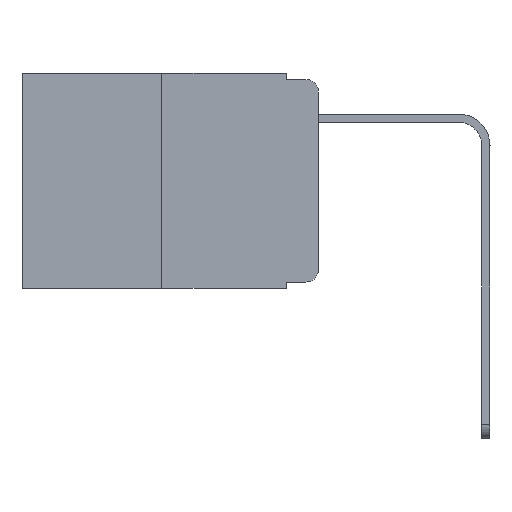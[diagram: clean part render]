
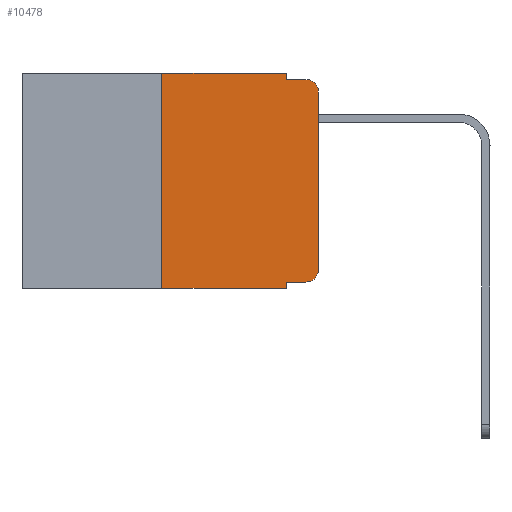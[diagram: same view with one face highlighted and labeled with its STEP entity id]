
A CAD part, left-side view. The second image highlights one B-rep face of the part: STEP entity #10478.
In plain terms, the highlighted planar face has unit normal (-1, 0, 0).
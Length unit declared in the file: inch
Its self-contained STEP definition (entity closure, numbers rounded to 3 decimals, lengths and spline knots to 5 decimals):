
#91 = VERTEX_POINT ( 'NONE', #7067 ) ;
#292 = CARTESIAN_POINT ( 'NONE',  ( 0., 0.25, 0. ) ) ;
#406 = LINE ( 'NONE', #9461, #6732 ) ;
#612 = DIRECTION ( 'NONE',  ( 0., -1., 0. ) ) ;
#641 = ORIENTED_EDGE ( 'NONE', *, *, #7964, .F. ) ;
#962 = EDGE_CURVE ( 'NONE', #13038, #2491, #13460, .T. ) ;
#1041 = EDGE_CURVE ( 'NONE', #91, #13038, #13301, .T. ) ;
#1203 = DIRECTION ( 'NONE',  ( 0., 0., 1. ) ) ;
#1241 = VECTOR ( 'NONE', #11664, 39.37008 ) ;
#1297 = DIRECTION ( 'NONE',  ( 0., 0., -1. ) ) ;
#1613 = VECTOR ( 'NONE', #12082, 39.37008 ) ;
#1673 = ORIENTED_EDGE ( 'NONE', *, *, #12184, .T. ) ;
#1841 = VERTEX_POINT ( 'NONE', #10940 ) ;
#2083 = LINE ( 'NONE', #6986, #6258 ) ;
#2445 = VERTEX_POINT ( 'NONE', #3387 ) ;
#2490 = DIRECTION ( 'NONE',  ( 0., 0., -1. ) ) ;
#2491 = VERTEX_POINT ( 'NONE', #6787 ) ;
#2557 = CARTESIAN_POINT ( 'NONE',  ( 0., 0.02, -0.333 ) ) ;
#2802 = VECTOR ( 'NONE', #5198, 39.37008 ) ;
#2973 = CARTESIAN_POINT ( 'NONE',  ( 0., 0.051, 0. ) ) ;
#3045 = ORIENTED_EDGE ( 'NONE', *, *, #10489, .T. ) ;
#3101 = VECTOR ( 'NONE', #2490, 39.37008 ) ;
#3387 = CARTESIAN_POINT ( 'NONE',  ( 0., 0.051, -0.343 ) ) ;
#3602 = ORIENTED_EDGE ( 'NONE', *, *, #13327, .T. ) ;
#3613 = CIRCLE ( 'NONE', #4885, 0.02 ) ;
#3756 = VECTOR ( 'NONE', #10365, 39.37008 ) ;
#4124 = DIRECTION ( 'NONE',  ( 0., 0., 1. ) ) ;
#4350 = ORIENTED_EDGE ( 'NONE', *, *, #962, .F. ) ;
#4607 = DIRECTION ( 'NONE',  ( -1., 0., 0. ) ) ;
#4625 = AXIS2_PLACEMENT_3D ( 'NONE', #11057, #11157, #7944 ) ;
#4651 = CARTESIAN_POINT ( 'NONE',  ( 0., 0.25, 0. ) ) ;
#4885 = AXIS2_PLACEMENT_3D ( 'NONE', #7748, #10828, #1297 ) ;
#5175 = VERTEX_POINT ( 'NONE', #2557 ) ;
#5198 = DIRECTION ( 'NONE',  ( 0., -1., 0. ) ) ;
#5305 = VERTEX_POINT ( 'NONE', #8576 ) ;
#5349 = VERTEX_POINT ( 'NONE', #10925 ) ;
#5919 = CARTESIAN_POINT ( 'NONE',  ( 0., 0., -0.313 ) ) ;
#5934 = LINE ( 'NONE', #8931, #1613 ) ;
#6072 = AXIS2_PLACEMENT_3D ( 'NONE', #13096, #4607, #12996 ) ;
#6258 = VECTOR ( 'NONE', #612, 39.37008 ) ;
#6732 = VECTOR ( 'NONE', #4124, 39.37008 ) ;
#6758 = CARTESIAN_POINT ( 'NONE',  ( 0., 0.051, -0.01 ) ) ;
#6787 = CARTESIAN_POINT ( 'NONE',  ( 0., 0.051, 0. ) ) ;
#6897 = ORIENTED_EDGE ( 'NONE', *, *, #10337, .T. ) ;
#6986 = CARTESIAN_POINT ( 'NONE',  ( 0., 0.473, -0.343 ) ) ;
#7067 = CARTESIAN_POINT ( 'NONE',  ( 0., 0.25, -0.343 ) ) ;
#7298 = FACE_OUTER_BOUND ( 'NONE', #13647, .T. ) ;
#7341 = CARTESIAN_POINT ( 'NONE',  ( 0., 0.051, -0.01 ) ) ;
#7595 = CIRCLE ( 'NONE', #6072, 0.02 ) ;
#7690 = EDGE_CURVE ( 'NONE', #10163, #5305, #11460, .T. ) ;
#7748 = CARTESIAN_POINT ( 'NONE',  ( 0., 0.02, -0.313 ) ) ;
#7944 = DIRECTION ( 'NONE',  ( 0., 0., -1. ) ) ;
#7964 = EDGE_CURVE ( 'NONE', #1841, #2445, #13416, .T. ) ;
#8316 = EDGE_CURVE ( 'NONE', #91, #2445, #2083, .T. ) ;
#8576 = CARTESIAN_POINT ( 'NONE',  ( 0., 0.02, -0.01 ) ) ;
#8931 = CARTESIAN_POINT ( 'NONE',  ( 0., 0.051, -0.333 ) ) ;
#8974 = PLANE ( 'NONE',  #4625 ) ;
#9461 = CARTESIAN_POINT ( 'NONE',  ( 0., 0., 0. ) ) ;
#9640 = VERTEX_POINT ( 'NONE', #5919 ) ;
#10100 = ORIENTED_EDGE ( 'NONE', *, *, #7690, .F. ) ;
#10163 = VERTEX_POINT ( 'NONE', #6758 ) ;
#10337 = EDGE_CURVE ( 'NONE', #5175, #9640, #3613, .T. ) ;
#10365 = DIRECTION ( 'NONE',  ( 0., -1., 0. ) ) ;
#10478 = ADVANCED_FACE ( 'NONE', ( #7298 ), #8974, .F. ) ;
#10489 = EDGE_CURVE ( 'NONE', #1841, #5175, #5934, .T. ) ;
#10496 = VECTOR ( 'NONE', #1203, 39.37008 ) ;
#10828 = DIRECTION ( 'NONE',  ( -1., 0., 0. ) ) ;
#10925 = CARTESIAN_POINT ( 'NONE',  ( 0., 0., -0.03 ) ) ;
#10932 = CARTESIAN_POINT ( 'NONE',  ( 0., 0.051, 0. ) ) ;
#10940 = CARTESIAN_POINT ( 'NONE',  ( 0., 0.051, -0.333 ) ) ;
#11057 = CARTESIAN_POINT ( 'NONE',  ( 0., 0.473, 0. ) ) ;
#11157 = DIRECTION ( 'NONE',  ( 1., 0., 0. ) ) ;
#11460 = LINE ( 'NONE', #7341, #3756 ) ;
#11628 = ORIENTED_EDGE ( 'NONE', *, *, #8316, .T. ) ;
#11629 = CARTESIAN_POINT ( 'NONE',  ( 0., 0.473, 0. ) ) ;
#11664 = DIRECTION ( 'NONE',  ( 0., 0., -1. ) ) ;
#12082 = DIRECTION ( 'NONE',  ( 0., -1., 0. ) ) ;
#12184 = EDGE_CURVE ( 'NONE', #9640, #5349, #406, .T. ) ;
#12409 = LINE ( 'NONE', #2973, #1241 ) ;
#12996 = DIRECTION ( 'NONE',  ( 0., 0., -1. ) ) ;
#13038 = VERTEX_POINT ( 'NONE', #4651 ) ;
#13096 = CARTESIAN_POINT ( 'NONE',  ( 0., 0.02, -0.03 ) ) ;
#13298 = ORIENTED_EDGE ( 'NONE', *, *, #13728, .F. ) ;
#13301 = LINE ( 'NONE', #292, #10496 ) ;
#13327 = EDGE_CURVE ( 'NONE', #5349, #5305, #7595, .T. ) ;
#13344 = ORIENTED_EDGE ( 'NONE', *, *, #1041, .F. ) ;
#13416 = LINE ( 'NONE', #10932, #3101 ) ;
#13460 = LINE ( 'NONE', #11629, #2802 ) ;
#13647 = EDGE_LOOP ( 'NONE', ( #1673, #3602, #10100, #13298, #4350, #13344, #11628, #641, #3045, #6897 ) ) ;
#13728 = EDGE_CURVE ( 'NONE', #2491, #10163, #12409, .T. ) ;
